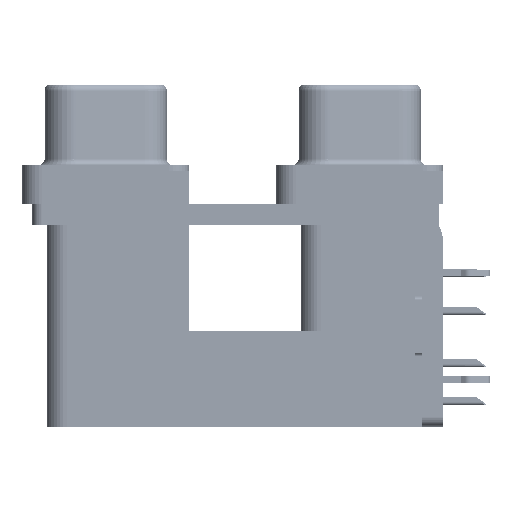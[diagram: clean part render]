
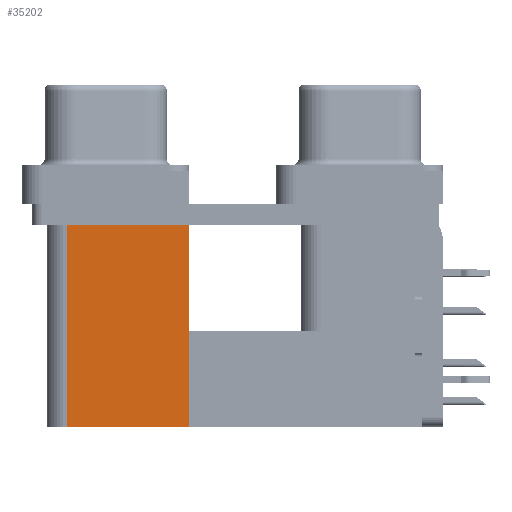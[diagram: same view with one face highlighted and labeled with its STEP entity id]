
A CAD part, left-side view. The second image highlights one B-rep face of the part: STEP entity #35202.
In plain terms, the highlighted planar face has unit normal (-1, 0, 0).
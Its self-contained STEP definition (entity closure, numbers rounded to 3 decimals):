
#145 = DIRECTION ( 'NONE',  ( 0., 0., 1. ) ) ;
#5099 = VERTEX_POINT ( 'NONE', #43881 ) ;
#8530 = DIRECTION ( 'NONE',  ( 0., 0., 1. ) ) ;
#9845 = AXIS2_PLACEMENT_3D ( 'NONE', #38804, #26914, #51229 ) ;
#12864 = CARTESIAN_POINT ( 'NONE',  ( 3.79, 21.975, -19.2 ) ) ;
#14959 = FACE_OUTER_BOUND ( 'NONE', #19862, .T. ) ;
#14982 = DIRECTION ( 'NONE',  ( 0., 1., 0. ) ) ;
#18693 = ORIENTED_EDGE ( 'NONE', *, *, #36814, .T. ) ;
#19862 = EDGE_LOOP ( 'NONE', ( #49639, #49758, #53031, #18693 ) ) ;
#22164 = VECTOR ( 'NONE', #22411, 1000. ) ;
#22411 = DIRECTION ( 'NONE',  ( 0., 1., 0. ) ) ;
#24800 = LINE ( 'NONE', #41279, #52305 ) ;
#26914 = DIRECTION ( 'NONE',  ( 1., 0., 0. ) ) ;
#27449 = PLANE ( 'NONE',  #9845 ) ;
#27473 = LINE ( 'NONE', #35568, #47131 ) ;
#29877 = VERTEX_POINT ( 'NONE', #35098 ) ;
#30352 = CARTESIAN_POINT ( 'NONE',  ( 3.79, 12.775, -2.5 ) ) ;
#31840 = EDGE_CURVE ( 'NONE', #5099, #29877, #27473, .T. ) ;
#33753 = VERTEX_POINT ( 'NONE', #41785 ) ;
#35098 = CARTESIAN_POINT ( 'NONE',  ( 3.79, 21.975, -19.2 ) ) ;
#35202 = ADVANCED_FACE ( 'NONE', ( #14959 ), #27449, .F. ) ;
#35568 = CARTESIAN_POINT ( 'NONE',  ( 3.79, 12.775, -19.2 ) ) ;
#36814 = EDGE_CURVE ( 'NONE', #5099, #41310, #24800, .T. ) ;
#37562 = EDGE_CURVE ( 'NONE', #41310, #33753, #52408, .T. ) ;
#38804 = CARTESIAN_POINT ( 'NONE',  ( 3.79, 12.775, -19.2 ) ) ;
#41279 = CARTESIAN_POINT ( 'NONE',  ( 3.79, 12.775, -19.2 ) ) ;
#41310 = VERTEX_POINT ( 'NONE', #30352 ) ;
#41785 = CARTESIAN_POINT ( 'NONE',  ( 3.79, 21.975, -2.5 ) ) ;
#42184 = VECTOR ( 'NONE', #8530, 1000. ) ;
#43881 = CARTESIAN_POINT ( 'NONE',  ( 3.79, 12.775, -19.2 ) ) ;
#47131 = VECTOR ( 'NONE', #14982, 1000. ) ;
#47282 = CARTESIAN_POINT ( 'NONE',  ( 3.79, 12.775, -2.5 ) ) ;
#49639 = ORIENTED_EDGE ( 'NONE', *, *, #37562, .T. ) ;
#49758 = ORIENTED_EDGE ( 'NONE', *, *, #51681, .F. ) ;
#51229 = DIRECTION ( 'NONE',  ( 0., 0., -1. ) ) ;
#51681 = EDGE_CURVE ( 'NONE', #29877, #33753, #53462, .T. ) ;
#52305 = VECTOR ( 'NONE', #145, 1000. ) ;
#52408 = LINE ( 'NONE', #47282, #22164 ) ;
#53031 = ORIENTED_EDGE ( 'NONE', *, *, #31840, .F. ) ;
#53462 = LINE ( 'NONE', #12864, #42184 ) ;
